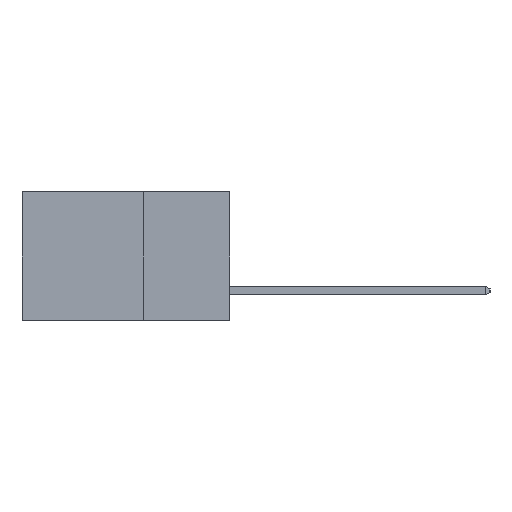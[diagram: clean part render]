
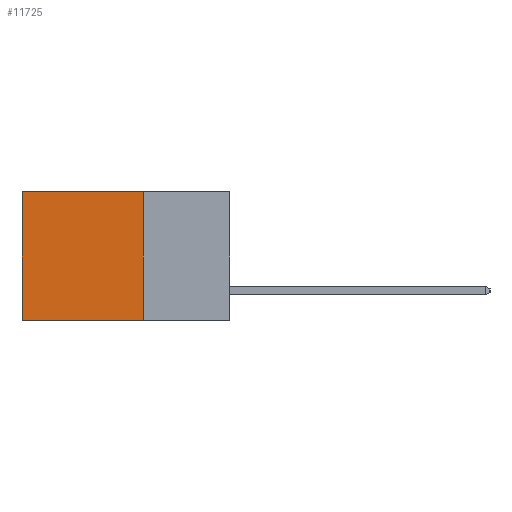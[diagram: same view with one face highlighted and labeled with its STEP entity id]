
A CAD part, left-side view. The second image highlights one B-rep face of the part: STEP entity #11725.
In plain terms, the highlighted planar face has unit normal (-1, 0, 0).
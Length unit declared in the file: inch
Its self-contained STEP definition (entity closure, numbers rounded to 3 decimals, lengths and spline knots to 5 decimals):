
#1748 = CARTESIAN_POINT ( 'NONE',  ( 0.2615, 0.25, 0. ) ) ;
#1850 = CARTESIAN_POINT ( 'NONE',  ( 0.2615, 0.6, 0. ) ) ;
#2074 = AXIS2_PLACEMENT_3D ( 'NONE', #13256, #5110, #16362 ) ;
#2558 = ORIENTED_EDGE ( 'NONE', *, *, #3824, .F. ) ;
#3235 = VERTEX_POINT ( 'NONE', #1748 ) ;
#3474 = PLANE ( 'NONE',  #2074 ) ;
#3568 = ORIENTED_EDGE ( 'NONE', *, *, #17078, .F. ) ;
#3824 = EDGE_CURVE ( 'NONE', #15545, #8696, #5426, .T. ) ;
#3835 = CARTESIAN_POINT ( 'NONE',  ( 0.2615, 0.25, -0.37 ) ) ;
#4526 = VECTOR ( 'NONE', #6155, 39.37008 ) ;
#5110 = DIRECTION ( 'NONE',  ( 1., 0., 0. ) ) ;
#5426 = LINE ( 'NONE', #19203, #17637 ) ;
#6155 = DIRECTION ( 'NONE',  ( 0., 1., 0. ) ) ;
#6671 = FACE_OUTER_BOUND ( 'NONE', #8811, .T. ) ;
#7724 = VECTOR ( 'NONE', #17157, 39.37008 ) ;
#8020 = DIRECTION ( 'NONE',  ( 0., 0., -1. ) ) ;
#8696 = VERTEX_POINT ( 'NONE', #14489 ) ;
#8729 = VECTOR ( 'NONE', #8020, 39.37008 ) ;
#8811 = EDGE_LOOP ( 'NONE', ( #9581, #2558, #3568, #9184 ) ) ;
#9184 = ORIENTED_EDGE ( 'NONE', *, *, #12746, .T. ) ;
#9239 = LINE ( 'NONE', #18925, #8729 ) ;
#9581 = ORIENTED_EDGE ( 'NONE', *, *, #17840, .T. ) ;
#10907 = CARTESIAN_POINT ( 'NONE',  ( 0.2615, 0.25, -0.37 ) ) ;
#11725 = ADVANCED_FACE ( 'NONE', ( #6671 ), #3474, .F. ) ;
#12746 = EDGE_CURVE ( 'NONE', #3235, #12954, #16373, .T. ) ;
#12954 = VERTEX_POINT ( 'NONE', #1850 ) ;
#13256 = CARTESIAN_POINT ( 'NONE',  ( 0.2615, 0.25, -0.37 ) ) ;
#14489 = CARTESIAN_POINT ( 'NONE',  ( 0.2615, 0.6, -0.37 ) ) ;
#15545 = VERTEX_POINT ( 'NONE', #3835 ) ;
#16362 = DIRECTION ( 'NONE',  ( 0., 0., -1. ) ) ;
#16373 = LINE ( 'NONE', #17295, #4526 ) ;
#17078 = EDGE_CURVE ( 'NONE', #3235, #15545, #20148, .T. ) ;
#17157 = DIRECTION ( 'NONE',  ( 0., 0., -1. ) ) ;
#17295 = CARTESIAN_POINT ( 'NONE',  ( 0.2615, 0.25, 0. ) ) ;
#17637 = VECTOR ( 'NONE', #19227, 39.37008 ) ;
#17840 = EDGE_CURVE ( 'NONE', #12954, #8696, #9239, .T. ) ;
#18925 = CARTESIAN_POINT ( 'NONE',  ( 0.2615, 0.6, -0.37 ) ) ;
#19203 = CARTESIAN_POINT ( 'NONE',  ( 0.2615, 0.25, -0.37 ) ) ;
#19227 = DIRECTION ( 'NONE',  ( 0., 1., 0. ) ) ;
#20148 = LINE ( 'NONE', #10907, #7724 ) ;
